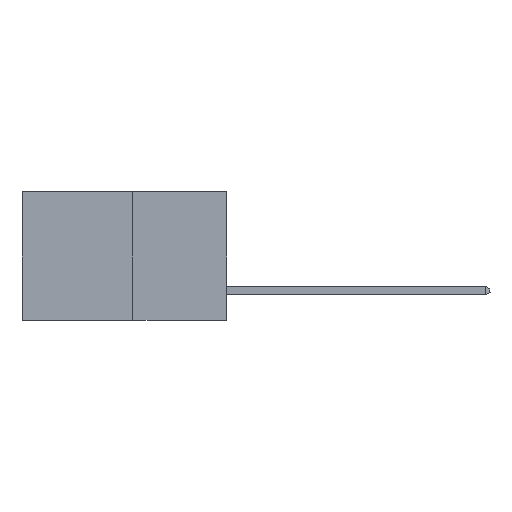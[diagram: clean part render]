
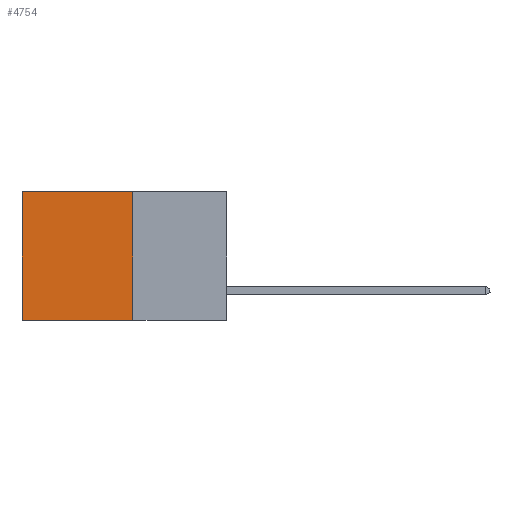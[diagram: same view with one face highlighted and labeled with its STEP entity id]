
A CAD part, left-side view. The second image highlights one B-rep face of the part: STEP entity #4754.
In plain terms, the highlighted planar face has unit normal (-1, 0, 0).
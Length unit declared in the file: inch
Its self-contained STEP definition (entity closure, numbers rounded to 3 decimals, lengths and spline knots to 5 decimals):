
#383 = VECTOR ( 'NONE', #23621, 39.37008 ) ;
#1298 = EDGE_CURVE ( 'NONE', #7802, #3654, #18474, .T. ) ;
#1350 = VERTEX_POINT ( 'NONE', #13470 ) ;
#2008 = LINE ( 'NONE', #15514, #23206 ) ;
#3248 = EDGE_CURVE ( 'NONE', #3654, #13017, #16746, .T. ) ;
#3654 = VERTEX_POINT ( 'NONE', #9131 ) ;
#4754 = ADVANCED_FACE ( 'NONE', ( #12632 ), #18187, .F. ) ;
#6352 = CARTESIAN_POINT ( 'NONE',  ( 0.277, 0.27, 0. ) ) ;
#6798 = DIRECTION ( 'NONE',  ( 0., 1., 0. ) ) ;
#7401 = DIRECTION ( 'NONE',  ( 0., 0., -1. ) ) ;
#7802 = VERTEX_POINT ( 'NONE', #22300 ) ;
#7997 = ORIENTED_EDGE ( 'NONE', *, *, #11059, .F. ) ;
#9131 = CARTESIAN_POINT ( 'NONE',  ( 0.277, 0.59, 0. ) ) ;
#9538 = AXIS2_PLACEMENT_3D ( 'NONE', #17635, #17586, #17582 ) ;
#11059 = EDGE_CURVE ( 'NONE', #7802, #1350, #2008, .T. ) ;
#12632 = FACE_OUTER_BOUND ( 'NONE', #19900, .T. ) ;
#12669 = DIRECTION ( 'NONE',  ( 0., 1., 0. ) ) ;
#13017 = VERTEX_POINT ( 'NONE', #15785 ) ;
#13470 = CARTESIAN_POINT ( 'NONE',  ( 0.277, 0.27, -0.37 ) ) ;
#15514 = CARTESIAN_POINT ( 'NONE',  ( 0.277, 0.27, -0.37 ) ) ;
#15785 = CARTESIAN_POINT ( 'NONE',  ( 0.277, 0.59, -0.37 ) ) ;
#16746 = LINE ( 'NONE', #21427, #383 ) ;
#16794 = ORIENTED_EDGE ( 'NONE', *, *, #1298, .T. ) ;
#17582 = DIRECTION ( 'NONE',  ( 0., 0., -1. ) ) ;
#17586 = DIRECTION ( 'NONE',  ( 1., 0., 0. ) ) ;
#17635 = CARTESIAN_POINT ( 'NONE',  ( 0.277, 0.27, -0.37 ) ) ;
#18187 = PLANE ( 'NONE',  #9538 ) ;
#18474 = LINE ( 'NONE', #6352, #23298 ) ;
#19900 = EDGE_LOOP ( 'NONE', ( #20539, #20670, #7997, #16794 ) ) ;
#20539 = ORIENTED_EDGE ( 'NONE', *, *, #3248, .T. ) ;
#20670 = ORIENTED_EDGE ( 'NONE', *, *, #20951, .F. ) ;
#20951 = EDGE_CURVE ( 'NONE', #1350, #13017, #21363, .T. ) ;
#21363 = LINE ( 'NONE', #22900, #26082 ) ;
#21427 = CARTESIAN_POINT ( 'NONE',  ( 0.277, 0.59, -0.37 ) ) ;
#22300 = CARTESIAN_POINT ( 'NONE',  ( 0.277, 0.27, 0. ) ) ;
#22900 = CARTESIAN_POINT ( 'NONE',  ( 0.277, 0.27, -0.37 ) ) ;
#23206 = VECTOR ( 'NONE', #7401, 39.37008 ) ;
#23298 = VECTOR ( 'NONE', #6798, 39.37008 ) ;
#23621 = DIRECTION ( 'NONE',  ( 0., 0., -1. ) ) ;
#26082 = VECTOR ( 'NONE', #12669, 39.37008 ) ;
